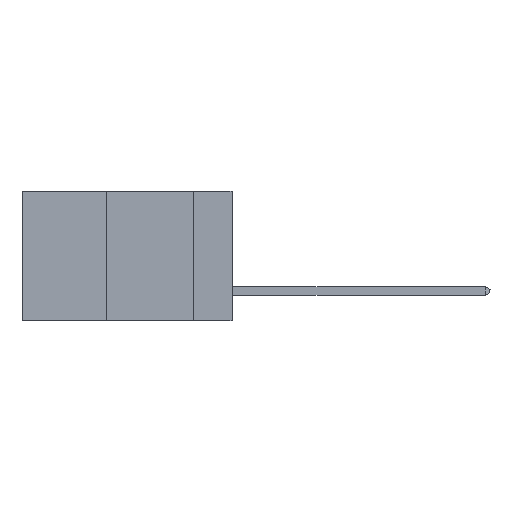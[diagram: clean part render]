
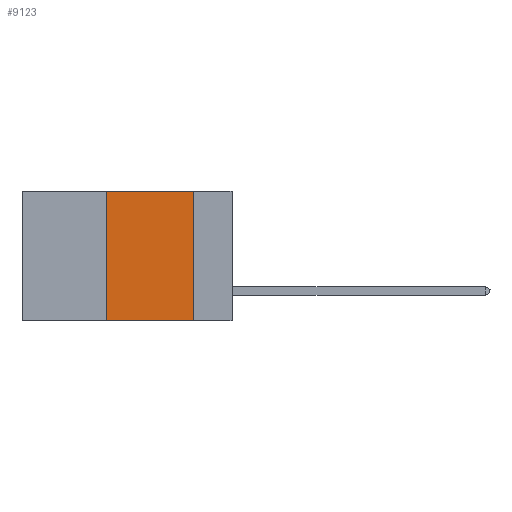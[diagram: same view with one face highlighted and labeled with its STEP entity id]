
A CAD part, left-side view. The second image highlights one B-rep face of the part: STEP entity #9123.
In plain terms, the highlighted planar face has unit normal (-1, 0, 0).
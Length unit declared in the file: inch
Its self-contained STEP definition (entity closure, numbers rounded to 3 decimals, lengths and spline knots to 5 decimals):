
#404 = DIRECTION ( 'NONE',  ( 0., -1., 0. ) ) ;
#439 = CARTESIAN_POINT ( 'NONE',  ( 0., 0.11, 0. ) ) ;
#652 = VERTEX_POINT ( 'NONE', #13312 ) ;
#912 = EDGE_CURVE ( 'NONE', #11703, #11624, #3081, .T. ) ;
#1388 = ORIENTED_EDGE ( 'NONE', *, *, #16645, .F. ) ;
#2053 = PLANE ( 'NONE',  #4695 ) ;
#3050 = LINE ( 'NONE', #11935, #9154 ) ;
#3081 = LINE ( 'NONE', #8444, #12804 ) ;
#3084 = LINE ( 'NONE', #439, #9856 ) ;
#3198 = CARTESIAN_POINT ( 'NONE',  ( 0., 0.6, 0. ) ) ;
#3491 = VECTOR ( 'NONE', #10352, 39.37008 ) ;
#3524 = VERTEX_POINT ( 'NONE', #9184 ) ;
#4695 = AXIS2_PLACEMENT_3D ( 'NONE', #3198, #12651, #7238 ) ;
#5304 = ORIENTED_EDGE ( 'NONE', *, *, #6072, .T. ) ;
#6072 = EDGE_CURVE ( 'NONE', #3524, #652, #3050, .T. ) ;
#6432 = DIRECTION ( 'NONE',  ( 0., -1., 0. ) ) ;
#7238 = DIRECTION ( 'NONE',  ( 0., 0., -1. ) ) ;
#7273 = LINE ( 'NONE', #17468, #3491 ) ;
#8241 = CARTESIAN_POINT ( 'NONE',  ( 0., 0.36, 0. ) ) ;
#8444 = CARTESIAN_POINT ( 'NONE',  ( 0., 0.6, 0. ) ) ;
#9123 = ADVANCED_FACE ( 'NONE', ( #12631 ), #2053, .F. ) ;
#9154 = VECTOR ( 'NONE', #6432, 39.37008 ) ;
#9184 = CARTESIAN_POINT ( 'NONE',  ( 0., 0.36, -0.37 ) ) ;
#9856 = VECTOR ( 'NONE', #11163, 39.37008 ) ;
#10352 = DIRECTION ( 'NONE',  ( 0., 0., 1. ) ) ;
#11163 = DIRECTION ( 'NONE',  ( 0., 0., -1. ) ) ;
#11624 = VERTEX_POINT ( 'NONE', #15098 ) ;
#11703 = VERTEX_POINT ( 'NONE', #8241 ) ;
#11935 = CARTESIAN_POINT ( 'NONE',  ( 0., 0.6, -0.37 ) ) ;
#12631 = FACE_OUTER_BOUND ( 'NONE', #13923, .T. ) ;
#12651 = DIRECTION ( 'NONE',  ( 1., 0., 0. ) ) ;
#12804 = VECTOR ( 'NONE', #404, 39.37008 ) ;
#13312 = CARTESIAN_POINT ( 'NONE',  ( 0., 0.11, -0.37 ) ) ;
#13923 = EDGE_LOOP ( 'NONE', ( #1388, #14504, #15901, #5304 ) ) ;
#14504 = ORIENTED_EDGE ( 'NONE', *, *, #912, .F. ) ;
#15098 = CARTESIAN_POINT ( 'NONE',  ( 0., 0.11, 0. ) ) ;
#15901 = ORIENTED_EDGE ( 'NONE', *, *, #16821, .F. ) ;
#16645 = EDGE_CURVE ( 'NONE', #11624, #652, #3084, .T. ) ;
#16821 = EDGE_CURVE ( 'NONE', #3524, #11703, #7273, .T. ) ;
#17468 = CARTESIAN_POINT ( 'NONE',  ( 0., 0.36, 0. ) ) ;
